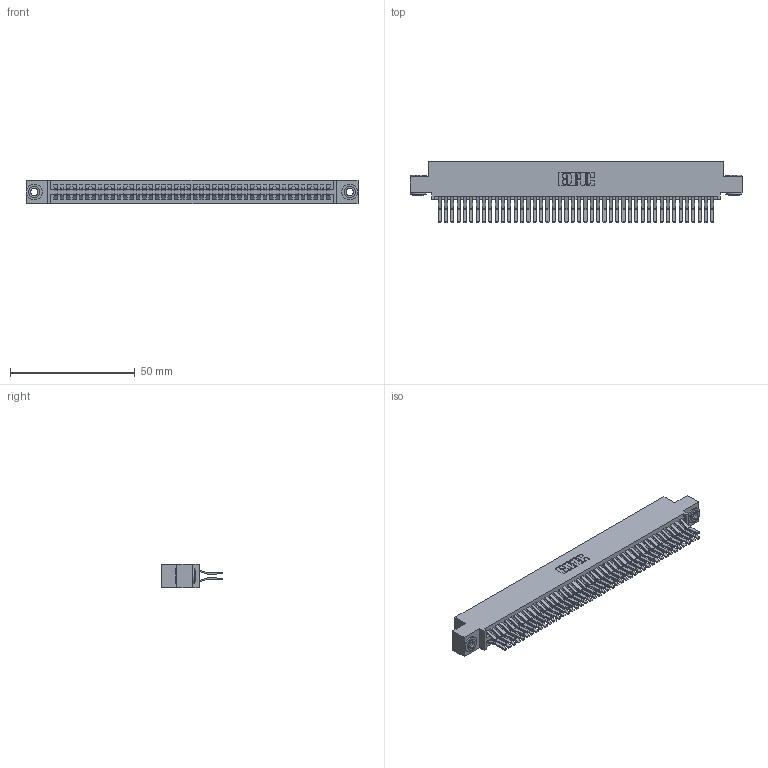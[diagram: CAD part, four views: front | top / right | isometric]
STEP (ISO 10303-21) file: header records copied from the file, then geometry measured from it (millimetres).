
FILE_DESCRIPTION (( 'STEP AP203' ), '1' );
FILE_NAME ('345-088-560-503.STEP', '2018-10-04T15:27:32', ( '' ), ( '' ), 'SwSTEP 2.0', 'SolidWorks 2016', '' );
FILE_SCHEMA (( 'CONFIG_CONTROL_DESIGN' ));
Length unit declared in the file: inch
Products named in the file (4): 345-292-001_560 Tail; 345-250-002_345-250-002-102; 345 Part_0.110 Offset - 0.156 Dia-TH; 345-088-560-503
Assembly tree (91 placements, depth 2):
  345-088-560-503
    345 Part_0.110 Offset - 0.156 Dia-TH
    345-292-001_560 Tail  x88
    345-250-002_345-250-002-102  x2
Bounding box: 132.97 x 24.45 x 9.4 mm (x, y, z)
Volume: 13458.1 mm3; surface area: 21713.3 mm2
Topology: 91 solids, 91 shells, 4744 faces, 14069 edges, 9258 vertices
Faces by surface type: plane 2998, cylinder 1738, cone 8
Entity records: 35124 total; most frequent: CARTESIAN_POINT 5863, ORIENTED_EDGE 5790, DIRECTION 5201, EDGE_CURVE 2895, VECTOR 2559, LINE 2559, VERTEX_POINT 1926, AXIS2_PLACEMENT_3D 1321
